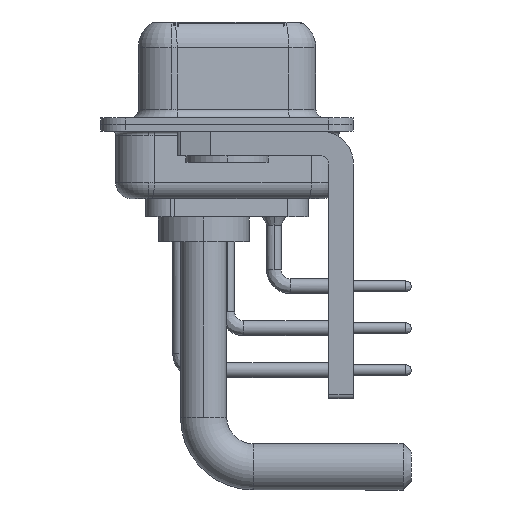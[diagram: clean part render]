
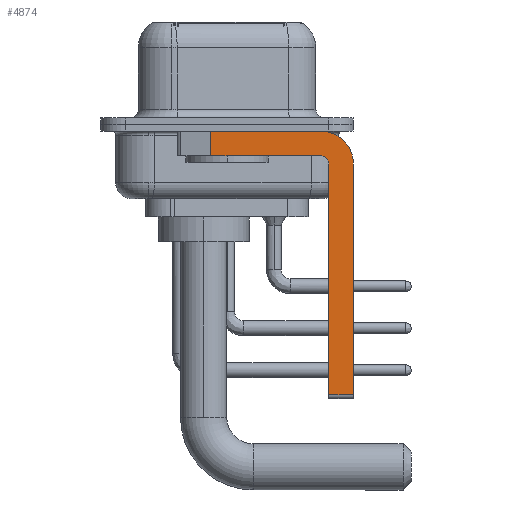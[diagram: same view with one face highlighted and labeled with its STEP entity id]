
A CAD part, left-side view. The second image highlights one B-rep face of the part: STEP entity #4874.
In plain terms, the highlighted planar face has unit normal (-1, 0, 0).
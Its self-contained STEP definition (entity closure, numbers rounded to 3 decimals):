
#487 = LINE ( 'NONE', #11729, #24306 ) ;
#562 = AXIS2_PLACEMENT_3D ( 'NONE', #20349, #26783, #20074 ) ;
#804 = VECTOR ( 'NONE', #11590, 1000. ) ;
#1980 = CARTESIAN_POINT ( 'NONE',  ( -2.9, -5.65, -1.9 ) ) ;
#2173 = CARTESIAN_POINT ( 'NONE',  ( -2.9, -6.15, -16.35 ) ) ;
#2463 = VERTEX_POINT ( 'NONE', #28801 ) ;
#2703 = LINE ( 'NONE', #11966, #5935 ) ;
#2746 = EDGE_CURVE ( 'NONE', #12239, #20121, #10150, .T. ) ;
#3305 = DIRECTION ( 'NONE',  ( 0., 0., -1. ) ) ;
#3604 = EDGE_CURVE ( 'NONE', #8160, #28872, #487, .T. ) ;
#3743 = DIRECTION ( 'NONE',  ( 0., 0., -1. ) ) ;
#3790 = CIRCLE ( 'NONE', #20820, 2. ) ;
#4460 = LINE ( 'NONE', #18464, #804 ) ;
#4874 = ADVANCED_FACE ( 'NONE', ( #10881 ), #6606, .F. ) ;
#5045 = EDGE_CURVE ( 'NONE', #8160, #11047, #18638, .T. ) ;
#5091 = ORIENTED_EDGE ( 'NONE', *, *, #2746, .T. ) ;
#5935 = VECTOR ( 'NONE', #12126, 1000. ) ;
#6067 = VECTOR ( 'NONE', #23661, 1000. ) ;
#6606 = PLANE ( 'NONE',  #18094 ) ;
#7990 = CARTESIAN_POINT ( 'NONE',  ( -2.9, -5.65, -2.4 ) ) ;
#8160 = VERTEX_POINT ( 'NONE', #2173 ) ;
#8922 = VECTOR ( 'NONE', #13782, 1000. ) ;
#9971 = ORIENTED_EDGE ( 'NONE', *, *, #25373, .F. ) ;
#10150 = LINE ( 'NONE', #12588, #20734 ) ;
#10881 = FACE_OUTER_BOUND ( 'NONE', #20381, .T. ) ;
#11047 = VERTEX_POINT ( 'NONE', #23145 ) ;
#11590 = DIRECTION ( 'NONE',  ( 0., -1., 0. ) ) ;
#11729 = CARTESIAN_POINT ( 'NONE',  ( -2.9, -6.15, -16.6 ) ) ;
#11966 = CARTESIAN_POINT ( 'NONE',  ( -2.9, -7.65, -2.4 ) ) ;
#12126 = DIRECTION ( 'NONE',  ( 0., 0., -1. ) ) ;
#12239 = VERTEX_POINT ( 'NONE', #16726 ) ;
#12310 = CARTESIAN_POINT ( 'NONE',  ( -2.9, -6.15, -2.4 ) ) ;
#12588 = CARTESIAN_POINT ( 'NONE',  ( -2.9, 0.978, -1.9 ) ) ;
#13179 = CARTESIAN_POINT ( 'NONE',  ( -2.9, -5.65, -2.4 ) ) ;
#13782 = DIRECTION ( 'NONE',  ( 0., 1., 0. ) ) ;
#15309 = DIRECTION ( 'NONE',  ( 1., 0., 0. ) ) ;
#15912 = CARTESIAN_POINT ( 'NONE',  ( -2.9, -5.65, -1.9 ) ) ;
#15944 = EDGE_CURVE ( 'NONE', #12239, #2463, #4460, .T. ) ;
#16726 = CARTESIAN_POINT ( 'NONE',  ( -2.9, 0.978, -0.4 ) ) ;
#17887 = CARTESIAN_POINT ( 'NONE',  ( -2.9, -7.65, -2.4 ) ) ;
#18094 = AXIS2_PLACEMENT_3D ( 'NONE', #13179, #15309, #3743 ) ;
#18464 = CARTESIAN_POINT ( 'NONE',  ( -2.9, 3., -0.4 ) ) ;
#18486 = VERTEX_POINT ( 'NONE', #1980 ) ;
#18638 = LINE ( 'NONE', #28086, #6067 ) ;
#19047 = DIRECTION ( 'NONE',  ( 0., 0., 1. ) ) ;
#19107 = ORIENTED_EDGE ( 'NONE', *, *, #22996, .F. ) ;
#19200 = EDGE_CURVE ( 'NONE', #2463, #21645, #3790, .T. ) ;
#19430 = DIRECTION ( 'NONE',  ( 0., 0., -1. ) ) ;
#20046 = ORIENTED_EDGE ( 'NONE', *, *, #19200, .F. ) ;
#20074 = DIRECTION ( 'NONE',  ( 0., 0., 1. ) ) ;
#20121 = VERTEX_POINT ( 'NONE', #22378 ) ;
#20349 = CARTESIAN_POINT ( 'NONE',  ( -2.9, -5.65, -2.4 ) ) ;
#20381 = EDGE_LOOP ( 'NONE', ( #25833, #5091, #9971, #19107, #23828, #26460, #21567, #20046 ) ) ;
#20734 = VECTOR ( 'NONE', #3305, 1000. ) ;
#20800 = LINE ( 'NONE', #15912, #8922 ) ;
#20820 = AXIS2_PLACEMENT_3D ( 'NONE', #7990, #24149, #19430 ) ;
#21567 = ORIENTED_EDGE ( 'NONE', *, *, #22853, .F. ) ;
#21645 = VERTEX_POINT ( 'NONE', #17887 ) ;
#22378 = CARTESIAN_POINT ( 'NONE',  ( -2.9, 0.978, -1.9 ) ) ;
#22853 = EDGE_CURVE ( 'NONE', #21645, #11047, #2703, .T. ) ;
#22996 = EDGE_CURVE ( 'NONE', #28872, #18486, #23874, .T. ) ;
#23145 = CARTESIAN_POINT ( 'NONE',  ( -2.9, -7.65, -16.35 ) ) ;
#23661 = DIRECTION ( 'NONE',  ( 0., -1., 0. ) ) ;
#23828 = ORIENTED_EDGE ( 'NONE', *, *, #3604, .F. ) ;
#23874 = CIRCLE ( 'NONE', #562, 0.5 ) ;
#24149 = DIRECTION ( 'NONE',  ( 1., 0., 0. ) ) ;
#24306 = VECTOR ( 'NONE', #19047, 1000. ) ;
#25373 = EDGE_CURVE ( 'NONE', #18486, #20121, #20800, .T. ) ;
#25833 = ORIENTED_EDGE ( 'NONE', *, *, #15944, .F. ) ;
#26460 = ORIENTED_EDGE ( 'NONE', *, *, #5045, .T. ) ;
#26783 = DIRECTION ( 'NONE',  ( -1., 0., 0. ) ) ;
#28086 = CARTESIAN_POINT ( 'NONE',  ( -2.9, -5.65, -16.35 ) ) ;
#28801 = CARTESIAN_POINT ( 'NONE',  ( -2.9, -5.65, -0.4 ) ) ;
#28872 = VERTEX_POINT ( 'NONE', #12310 ) ;
